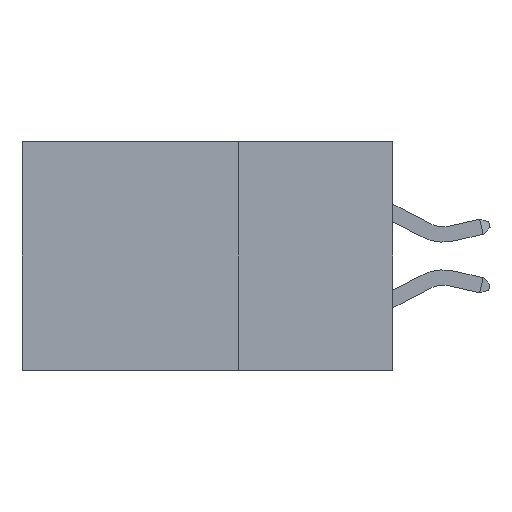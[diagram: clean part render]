
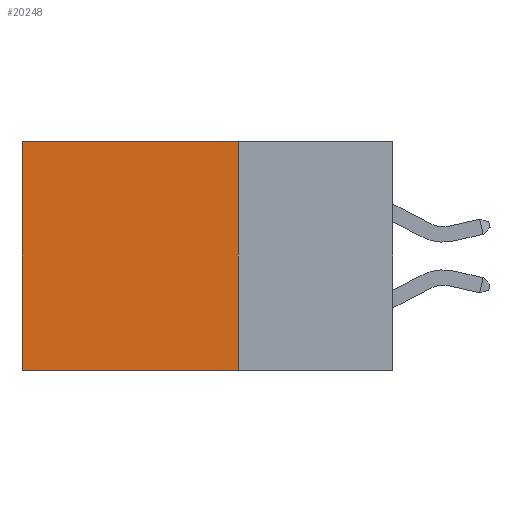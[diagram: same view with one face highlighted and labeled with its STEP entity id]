
A CAD part, left-side view. The second image highlights one B-rep face of the part: STEP entity #20248.
In plain terms, the highlighted planar face has unit normal (-1, 0, 0).
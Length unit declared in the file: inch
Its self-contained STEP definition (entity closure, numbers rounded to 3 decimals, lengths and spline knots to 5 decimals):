
#661 = VECTOR ( 'NONE', #27678, 39.37008 ) ;
#1529 = DIRECTION ( 'NONE',  ( 0., 1., 0. ) ) ;
#2110 = CARTESIAN_POINT ( 'NONE',  ( 0.2875, 0.25, -0.37 ) ) ;
#2904 = PLANE ( 'NONE',  #16281 ) ;
#3648 = VECTOR ( 'NONE', #1529, 39.37008 ) ;
#5580 = EDGE_LOOP ( 'NONE', ( #36434, #22189, #15394, #12347 ) ) ;
#7286 = CARTESIAN_POINT ( 'NONE',  ( 0.2875, 0.25, 0. ) ) ;
#9591 = CARTESIAN_POINT ( 'NONE',  ( 0.2875, 0.6, 0. ) ) ;
#11156 = EDGE_CURVE ( 'NONE', #14257, #18665, #31539, .T. ) ;
#11465 = CARTESIAN_POINT ( 'NONE',  ( 0.2875, 0.25, 0. ) ) ;
#12193 = LINE ( 'NONE', #9591, #28961 ) ;
#12347 = ORIENTED_EDGE ( 'NONE', *, *, #13769, .T. ) ;
#13382 = CARTESIAN_POINT ( 'NONE',  ( 0.2875, 0.25, -0.37 ) ) ;
#13769 = EDGE_CURVE ( 'NONE', #26963, #35199, #29710, .T. ) ;
#13839 = CARTESIAN_POINT ( 'NONE',  ( 0.2875, 0.6, -0.37 ) ) ;
#14257 = VERTEX_POINT ( 'NONE', #13382 ) ;
#15394 = ORIENTED_EDGE ( 'NONE', *, *, #15406, .F. ) ;
#15406 = EDGE_CURVE ( 'NONE', #26963, #14257, #17892, .T. ) ;
#16281 = AXIS2_PLACEMENT_3D ( 'NONE', #11465, #22865, #20037 ) ;
#17892 = LINE ( 'NONE', #24252, #24591 ) ;
#18442 = DIRECTION ( 'NONE',  ( 0., 0., -1. ) ) ;
#18665 = VERTEX_POINT ( 'NONE', #13839 ) ;
#19274 = CARTESIAN_POINT ( 'NONE',  ( 0.2875, 0.25, 0. ) ) ;
#20037 = DIRECTION ( 'NONE',  ( 0., 0., -1. ) ) ;
#20248 = ADVANCED_FACE ( 'NONE', ( #24385 ), #2904, .F. ) ;
#22189 = ORIENTED_EDGE ( 'NONE', *, *, #11156, .F. ) ;
#22865 = DIRECTION ( 'NONE',  ( 1., 0., 0. ) ) ;
#24252 = CARTESIAN_POINT ( 'NONE',  ( 0.2875, 0.25, 0. ) ) ;
#24385 = FACE_OUTER_BOUND ( 'NONE', #5580, .T. ) ;
#24407 = EDGE_CURVE ( 'NONE', #35199, #18665, #12193, .T. ) ;
#24591 = VECTOR ( 'NONE', #18442, 39.37008 ) ;
#26045 = DIRECTION ( 'NONE',  ( 0., 0., -1. ) ) ;
#26963 = VERTEX_POINT ( 'NONE', #19274 ) ;
#27678 = DIRECTION ( 'NONE',  ( 0., 1., 0. ) ) ;
#28961 = VECTOR ( 'NONE', #26045, 39.37008 ) ;
#29710 = LINE ( 'NONE', #7286, #3648 ) ;
#31539 = LINE ( 'NONE', #2110, #661 ) ;
#33965 = CARTESIAN_POINT ( 'NONE',  ( 0.2875, 0.6, 0. ) ) ;
#35199 = VERTEX_POINT ( 'NONE', #33965 ) ;
#36434 = ORIENTED_EDGE ( 'NONE', *, *, #24407, .T. ) ;
